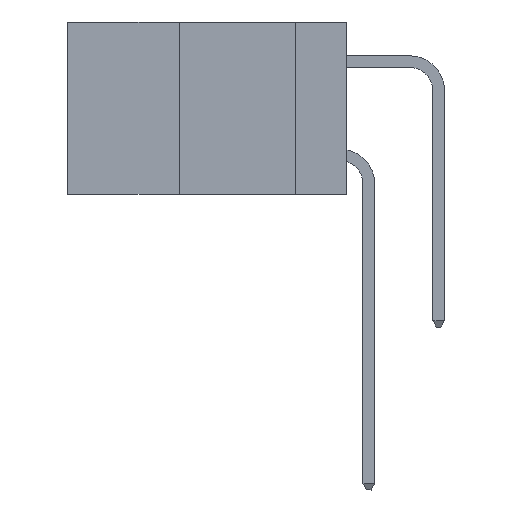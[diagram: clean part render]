
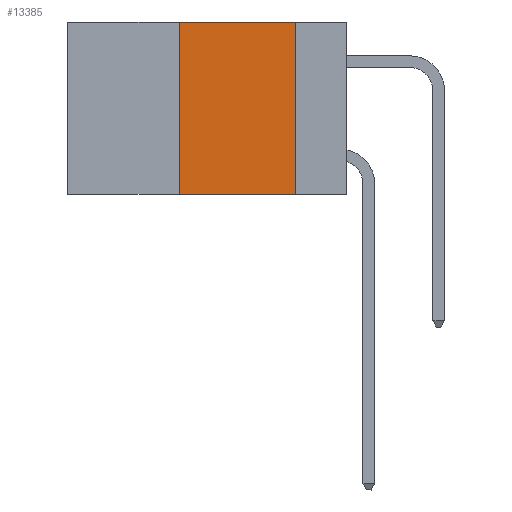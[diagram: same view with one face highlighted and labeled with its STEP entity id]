
A CAD part, left-side view. The second image highlights one B-rep face of the part: STEP entity #13385.
In plain terms, the highlighted planar face has unit normal (-1, 0, 0).
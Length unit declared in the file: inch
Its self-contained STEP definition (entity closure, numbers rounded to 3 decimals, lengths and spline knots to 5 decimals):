
#153 = EDGE_CURVE ( 'NONE', #8415, #1380, #14187, .T. ) ;
#1112 = PLANE ( 'NONE',  #4366 ) ;
#1160 = DIRECTION ( 'NONE',  ( 0., 0., -1. ) ) ;
#1380 = VERTEX_POINT ( 'NONE', #9103 ) ;
#2195 = LINE ( 'NONE', #12901, #16254 ) ;
#2479 = VERTEX_POINT ( 'NONE', #5345 ) ;
#2919 = EDGE_CURVE ( 'NONE', #8415, #6808, #8371, .T. ) ;
#4366 = AXIS2_PLACEMENT_3D ( 'NONE', #7523, #7604, #12861 ) ;
#4627 = CARTESIAN_POINT ( 'NONE',  ( 0., 0.6, 0. ) ) ;
#4742 = ORIENTED_EDGE ( 'NONE', *, *, #16689, .F. ) ;
#5345 = CARTESIAN_POINT ( 'NONE',  ( 0., 0.11, 0. ) ) ;
#5811 = DIRECTION ( 'NONE',  ( 0., -1., 0. ) ) ;
#5850 = CARTESIAN_POINT ( 'NONE',  ( 0., 0.11, -0.37 ) ) ;
#5905 = LINE ( 'NONE', #4627, #11681 ) ;
#5940 = ORIENTED_EDGE ( 'NONE', *, *, #10296, .F. ) ;
#6366 = CARTESIAN_POINT ( 'NONE',  ( 0., 0.36, 0. ) ) ;
#6520 = CARTESIAN_POINT ( 'NONE',  ( 0., 0.36, -0.37 ) ) ;
#6808 = VERTEX_POINT ( 'NONE', #5850 ) ;
#7523 = CARTESIAN_POINT ( 'NONE',  ( 0., 0.6, 0. ) ) ;
#7604 = DIRECTION ( 'NONE',  ( 1., 0., 0. ) ) ;
#8197 = DIRECTION ( 'NONE',  ( 0., -1., 0. ) ) ;
#8371 = LINE ( 'NONE', #16388, #12092 ) ;
#8415 = VERTEX_POINT ( 'NONE', #6520 ) ;
#9103 = CARTESIAN_POINT ( 'NONE',  ( 0., 0.36, 0. ) ) ;
#10296 = EDGE_CURVE ( 'NONE', #1380, #2479, #5905, .T. ) ;
#11681 = VECTOR ( 'NONE', #5811, 39.37008 ) ;
#11983 = ORIENTED_EDGE ( 'NONE', *, *, #2919, .T. ) ;
#12092 = VECTOR ( 'NONE', #8197, 39.37008 ) ;
#12861 = DIRECTION ( 'NONE',  ( 0., 0., -1. ) ) ;
#12901 = CARTESIAN_POINT ( 'NONE',  ( 0., 0.11, 0. ) ) ;
#13385 = ADVANCED_FACE ( 'NONE', ( #15203 ), #1112, .F. ) ;
#14187 = LINE ( 'NONE', #6366, #15928 ) ;
#14564 = EDGE_LOOP ( 'NONE', ( #4742, #5940, #16909, #11983 ) ) ;
#14774 = DIRECTION ( 'NONE',  ( 0., 0., 1. ) ) ;
#15203 = FACE_OUTER_BOUND ( 'NONE', #14564, .T. ) ;
#15928 = VECTOR ( 'NONE', #14774, 39.37008 ) ;
#16254 = VECTOR ( 'NONE', #1160, 39.37008 ) ;
#16388 = CARTESIAN_POINT ( 'NONE',  ( 0., 0.6, -0.37 ) ) ;
#16689 = EDGE_CURVE ( 'NONE', #2479, #6808, #2195, .T. ) ;
#16909 = ORIENTED_EDGE ( 'NONE', *, *, #153, .F. ) ;
